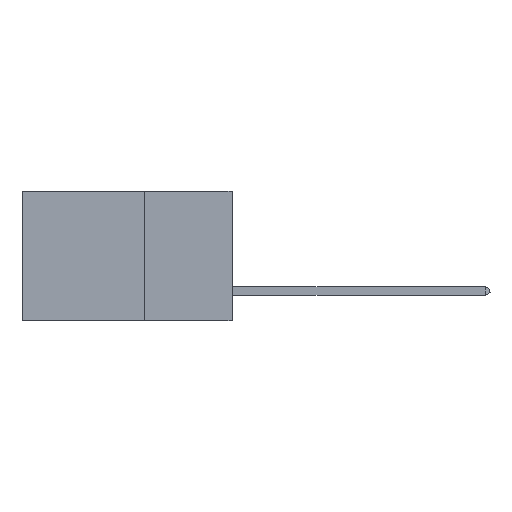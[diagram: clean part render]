
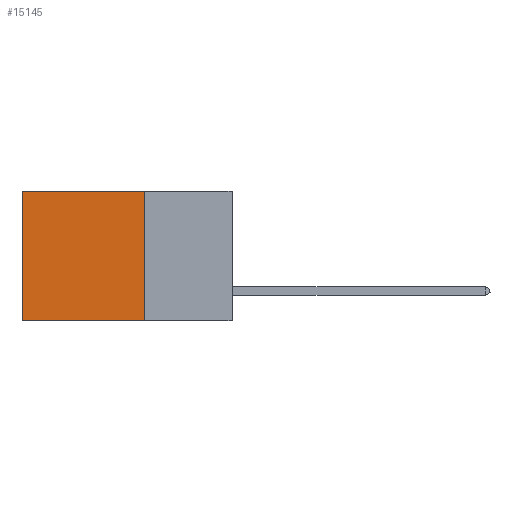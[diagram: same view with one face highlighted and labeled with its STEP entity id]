
A CAD part, left-side view. The second image highlights one B-rep face of the part: STEP entity #15145.
In plain terms, the highlighted planar face has unit normal (-1, 0, 0).
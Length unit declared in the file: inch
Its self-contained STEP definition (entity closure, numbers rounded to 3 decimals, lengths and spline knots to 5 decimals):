
#367 = EDGE_CURVE ( 'NONE', #428, #7030, #626, .T. ) ;
#428 = VERTEX_POINT ( 'NONE', #14254 ) ;
#429 = AXIS2_PLACEMENT_3D ( 'NONE', #17363, #12811, #6709 ) ;
#451 = LINE ( 'NONE', #13224, #9342 ) ;
#616 = DIRECTION ( 'NONE',  ( 0., 0., -1. ) ) ;
#626 = LINE ( 'NONE', #12326, #9053 ) ;
#1144 = CARTESIAN_POINT ( 'NONE',  ( 0.2875, 0.6, 0. ) ) ;
#1719 = FACE_OUTER_BOUND ( 'NONE', #2491, .T. ) ;
#2491 = EDGE_LOOP ( 'NONE', ( #2872, #13384, #14230, #9037 ) ) ;
#2872 = ORIENTED_EDGE ( 'NONE', *, *, #9932, .T. ) ;
#4204 = LINE ( 'NONE', #9055, #12157 ) ;
#4661 = EDGE_CURVE ( 'NONE', #428, #12952, #451, .T. ) ;
#6709 = DIRECTION ( 'NONE',  ( 0., 0., -1. ) ) ;
#7030 = VERTEX_POINT ( 'NONE', #10351 ) ;
#8508 = LINE ( 'NONE', #12344, #13600 ) ;
#9037 = ORIENTED_EDGE ( 'NONE', *, *, #4661, .T. ) ;
#9053 = VECTOR ( 'NONE', #616, 39.37008 ) ;
#9055 = CARTESIAN_POINT ( 'NONE',  ( 0.2875, 0.25, -0.37 ) ) ;
#9342 = VECTOR ( 'NONE', #14712, 39.37008 ) ;
#9932 = EDGE_CURVE ( 'NONE', #12952, #15177, #8508, .T. ) ;
#10351 = CARTESIAN_POINT ( 'NONE',  ( 0.2875, 0.25, -0.37 ) ) ;
#11438 = CARTESIAN_POINT ( 'NONE',  ( 0.2875, 0.6, -0.37 ) ) ;
#11824 = EDGE_CURVE ( 'NONE', #7030, #15177, #4204, .T. ) ;
#12157 = VECTOR ( 'NONE', #15035, 39.37008 ) ;
#12326 = CARTESIAN_POINT ( 'NONE',  ( 0.2875, 0.25, 0. ) ) ;
#12344 = CARTESIAN_POINT ( 'NONE',  ( 0.2875, 0.6, 0. ) ) ;
#12747 = PLANE ( 'NONE',  #429 ) ;
#12769 = DIRECTION ( 'NONE',  ( 0., 0., -1. ) ) ;
#12811 = DIRECTION ( 'NONE',  ( 1., 0., 0. ) ) ;
#12952 = VERTEX_POINT ( 'NONE', #1144 ) ;
#13224 = CARTESIAN_POINT ( 'NONE',  ( 0.2875, 0.25, 0. ) ) ;
#13384 = ORIENTED_EDGE ( 'NONE', *, *, #11824, .F. ) ;
#13600 = VECTOR ( 'NONE', #12769, 39.37008 ) ;
#14230 = ORIENTED_EDGE ( 'NONE', *, *, #367, .F. ) ;
#14254 = CARTESIAN_POINT ( 'NONE',  ( 0.2875, 0.25, 0. ) ) ;
#14712 = DIRECTION ( 'NONE',  ( 0., 1., 0. ) ) ;
#15035 = DIRECTION ( 'NONE',  ( 0., 1., 0. ) ) ;
#15145 = ADVANCED_FACE ( 'NONE', ( #1719 ), #12747, .F. ) ;
#15177 = VERTEX_POINT ( 'NONE', #11438 ) ;
#17363 = CARTESIAN_POINT ( 'NONE',  ( 0.2875, 0.25, 0. ) ) ;
